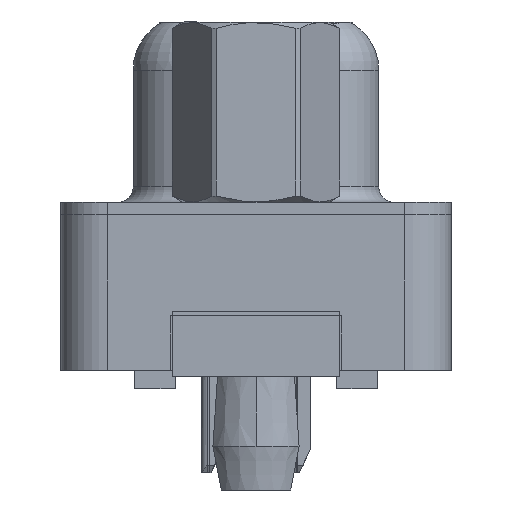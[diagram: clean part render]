
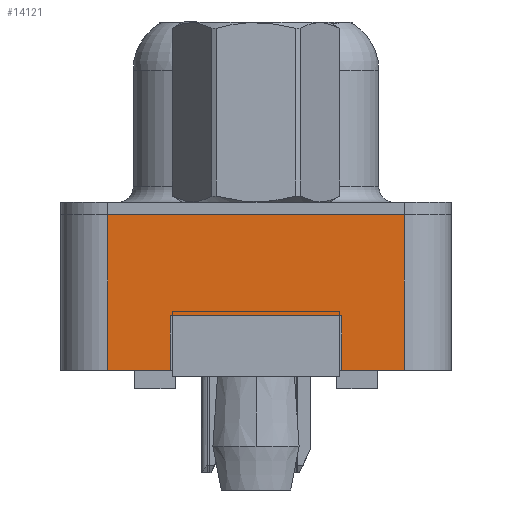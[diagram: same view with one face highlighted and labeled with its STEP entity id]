
A CAD part, left-side view. The second image highlights one B-rep face of the part: STEP entity #14121.
In plain terms, the highlighted planar face has unit normal (-1, 0, 0).
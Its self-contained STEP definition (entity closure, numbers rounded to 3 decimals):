
#592 = DIRECTION ( 'NONE',  ( 0., 0., 1. ) ) ;
#666 = AXIS2_PLACEMENT_3D ( 'NONE', #27265, #7578, #592 ) ;
#717 = LINE ( 'NONE', #13706, #13133 ) ;
#928 = DIRECTION ( 'NONE',  ( 0., -1., 0. ) ) ;
#944 = ORIENTED_EDGE ( 'NONE', *, *, #2961, .F. ) ;
#1190 = CARTESIAN_POINT ( 'NONE',  ( -2.91, 4.775, 0. ) ) ;
#2961 = EDGE_CURVE ( 'NONE', #25612, #22922, #11504, .T. ) ;
#3145 = FACE_OUTER_BOUND ( 'NONE', #27326, .T. ) ;
#3208 = CARTESIAN_POINT ( 'NONE',  ( -2.91, 2.75, -3.25 ) ) ;
#3576 = EDGE_CURVE ( 'NONE', #15865, #13166, #6649, .T. ) ;
#3952 = EDGE_CURVE ( 'NONE', #12281, #8892, #25165, .T. ) ;
#4499 = CARTESIAN_POINT ( 'NONE',  ( -2.91, -4.775, -5. ) ) ;
#4685 = CARTESIAN_POINT ( 'NONE',  ( -2.91, -2.75, -3.25 ) ) ;
#5286 = CARTESIAN_POINT ( 'NONE',  ( -2.91, -4.775, -5. ) ) ;
#5808 = VECTOR ( 'NONE', #17962, 1000. ) ;
#6119 = VECTOR ( 'NONE', #19071, 1000. ) ;
#6293 = ORIENTED_EDGE ( 'NONE', *, *, #25337, .T. ) ;
#6566 = EDGE_CURVE ( 'NONE', #25612, #20628, #6773, .T. ) ;
#6649 = LINE ( 'NONE', #4499, #9634 ) ;
#6773 = LINE ( 'NONE', #15476, #17307 ) ;
#7578 = DIRECTION ( 'NONE',  ( -1., 0., 0. ) ) ;
#8125 = ORIENTED_EDGE ( 'NONE', *, *, #13464, .T. ) ;
#8456 = VECTOR ( 'NONE', #9748, 1000. ) ;
#8892 = VERTEX_POINT ( 'NONE', #10523 ) ;
#8964 = DIRECTION ( 'NONE',  ( 0., 1., 0. ) ) ;
#9533 = CARTESIAN_POINT ( 'NONE',  ( -2.91, 4.775, -5. ) ) ;
#9634 = VECTOR ( 'NONE', #928, 1000. ) ;
#9748 = DIRECTION ( 'NONE',  ( 0., -1., 0. ) ) ;
#10073 = ORIENTED_EDGE ( 'NONE', *, *, #22402, .F. ) ;
#10391 = ORIENTED_EDGE ( 'NONE', *, *, #6566, .T. ) ;
#10486 = LINE ( 'NONE', #23336, #6119 ) ;
#10523 = CARTESIAN_POINT ( 'NONE',  ( -2.91, -4.775, 0. ) ) ;
#11101 = CARTESIAN_POINT ( 'NONE',  ( -2.91, 2.75, -5. ) ) ;
#11504 = LINE ( 'NONE', #24636, #27215 ) ;
#12281 = VERTEX_POINT ( 'NONE', #1190 ) ;
#12570 = LINE ( 'NONE', #27401, #17954 ) ;
#13000 = EDGE_CURVE ( 'NONE', #22922, #13166, #12570, .T. ) ;
#13133 = VECTOR ( 'NONE', #24401, 1000. ) ;
#13166 = VERTEX_POINT ( 'NONE', #11101 ) ;
#13464 = EDGE_CURVE ( 'NONE', #20628, #14065, #10486, .T. ) ;
#13706 = CARTESIAN_POINT ( 'NONE',  ( -2.91, -4.775, -5. ) ) ;
#13954 = LINE ( 'NONE', #18106, #5808 ) ;
#14065 = VERTEX_POINT ( 'NONE', #5286 ) ;
#14121 = ADVANCED_FACE ( 'NONE', ( #3145 ), #20570, .T. ) ;
#15069 = DIRECTION ( 'NONE',  ( 0., 0., -1. ) ) ;
#15476 = CARTESIAN_POINT ( 'NONE',  ( -2.91, -2.75, -3.25 ) ) ;
#15865 = VERTEX_POINT ( 'NONE', #9533 ) ;
#17307 = VECTOR ( 'NONE', #15069, 1000. ) ;
#17954 = VECTOR ( 'NONE', #23546, 1000. ) ;
#17962 = DIRECTION ( 'NONE',  ( 0., 0., 1. ) ) ;
#18106 = CARTESIAN_POINT ( 'NONE',  ( -2.91, 4.775, -5. ) ) ;
#18561 = ORIENTED_EDGE ( 'NONE', *, *, #3952, .F. ) ;
#18668 = ORIENTED_EDGE ( 'NONE', *, *, #3576, .T. ) ;
#19071 = DIRECTION ( 'NONE',  ( 0., -1., 0. ) ) ;
#20570 = PLANE ( 'NONE',  #666 ) ;
#20628 = VERTEX_POINT ( 'NONE', #26962 ) ;
#22402 = EDGE_CURVE ( 'NONE', #15865, #12281, #13954, .T. ) ;
#22922 = VERTEX_POINT ( 'NONE', #3208 ) ;
#23157 = CARTESIAN_POINT ( 'NONE',  ( -2.91, -4.775, 0. ) ) ;
#23336 = CARTESIAN_POINT ( 'NONE',  ( -2.91, -4.775, -5. ) ) ;
#23546 = DIRECTION ( 'NONE',  ( 0., 0., -1. ) ) ;
#24401 = DIRECTION ( 'NONE',  ( 0., 0., 1. ) ) ;
#24636 = CARTESIAN_POINT ( 'NONE',  ( -2.91, 2.75, -3.25 ) ) ;
#25165 = LINE ( 'NONE', #23157, #8456 ) ;
#25337 = EDGE_CURVE ( 'NONE', #14065, #8892, #717, .T. ) ;
#25612 = VERTEX_POINT ( 'NONE', #4685 ) ;
#26486 = ORIENTED_EDGE ( 'NONE', *, *, #13000, .F. ) ;
#26962 = CARTESIAN_POINT ( 'NONE',  ( -2.91, -2.75, -5. ) ) ;
#27215 = VECTOR ( 'NONE', #8964, 1000. ) ;
#27265 = CARTESIAN_POINT ( 'NONE',  ( -2.91, -4.775, -5. ) ) ;
#27326 = EDGE_LOOP ( 'NONE', ( #10391, #8125, #6293, #18561, #10073, #18668, #26486, #944 ) ) ;
#27401 = CARTESIAN_POINT ( 'NONE',  ( -2.91, 2.75, -3.25 ) ) ;
